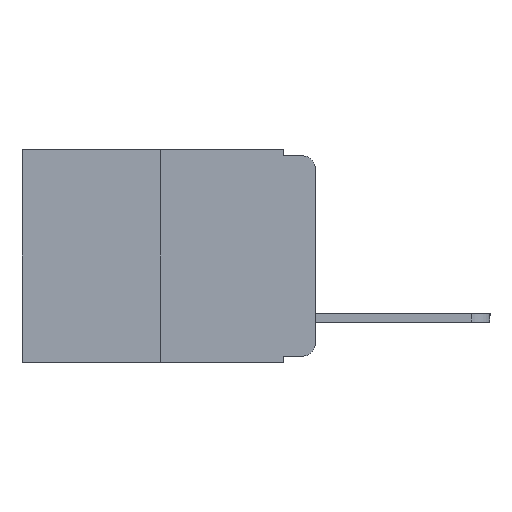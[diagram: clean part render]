
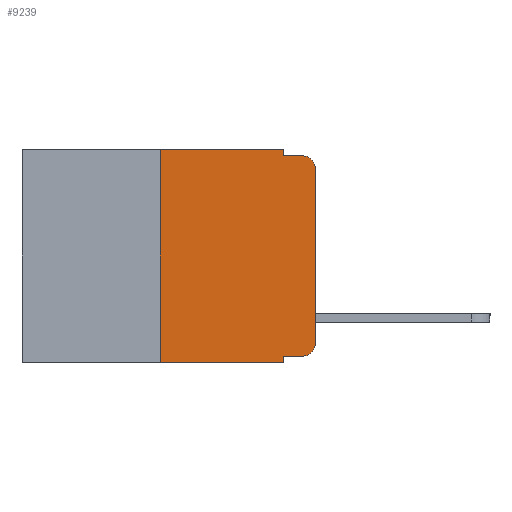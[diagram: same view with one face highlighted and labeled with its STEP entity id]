
A CAD part, left-side view. The second image highlights one B-rep face of the part: STEP entity #9239.
In plain terms, the highlighted planar face has unit normal (-1, 0, 0).
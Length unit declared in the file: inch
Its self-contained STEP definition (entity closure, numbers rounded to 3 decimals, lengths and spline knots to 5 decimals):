
#106 = CARTESIAN_POINT ( 'NONE',  ( 0., 0.473, 0. ) ) ;
#136 = DIRECTION ( 'NONE',  ( 0., 0., -1. ) ) ;
#495 = ORIENTED_EDGE ( 'NONE', *, *, #8389, .T. ) ;
#708 = CARTESIAN_POINT ( 'NONE',  ( 0., 0.02, -0.01 ) ) ;
#1027 = LINE ( 'NONE', #1408, #10063 ) ;
#1173 = DIRECTION ( 'NONE',  ( -1., 0., 0. ) ) ;
#1180 = VERTEX_POINT ( 'NONE', #7032 ) ;
#1190 = CARTESIAN_POINT ( 'NONE',  ( 0., 0.25, 0. ) ) ;
#1201 = CARTESIAN_POINT ( 'NONE',  ( 0., 0.02, -0.313 ) ) ;
#1278 = VERTEX_POINT ( 'NONE', #7676 ) ;
#1378 = CARTESIAN_POINT ( 'NONE',  ( 0., 0.02, -0.03 ) ) ;
#1408 = CARTESIAN_POINT ( 'NONE',  ( 0., 0.473, -0.343 ) ) ;
#1604 = CARTESIAN_POINT ( 'NONE',  ( 0., 0.051, -0.333 ) ) ;
#1689 = DIRECTION ( 'NONE',  ( 0., -1., 0. ) ) ;
#2374 = DIRECTION ( 'NONE',  ( 0., 0., -1. ) ) ;
#2413 = DIRECTION ( 'NONE',  ( 0., -1., 0. ) ) ;
#3088 = ORIENTED_EDGE ( 'NONE', *, *, #10665, .T. ) ;
#3316 = VERTEX_POINT ( 'NONE', #7626 ) ;
#3732 = LINE ( 'NONE', #106, #8022 ) ;
#3818 = EDGE_CURVE ( 'NONE', #10033, #6975, #5031, .T. ) ;
#3880 = CARTESIAN_POINT ( 'NONE',  ( 0., 0.051, -0.333 ) ) ;
#4171 = VERTEX_POINT ( 'NONE', #3880 ) ;
#4238 = DIRECTION ( 'NONE',  ( 0., 0., -1. ) ) ;
#4315 = VECTOR ( 'NONE', #7497, 39.37008 ) ;
#4344 = CARTESIAN_POINT ( 'NONE',  ( 0., 0.25, 0. ) ) ;
#4389 = AXIS2_PLACEMENT_3D ( 'NONE', #4956, #5806, #136 ) ;
#4413 = EDGE_CURVE ( 'NONE', #4171, #10033, #9331, .T. ) ;
#4479 = CARTESIAN_POINT ( 'NONE',  ( 0., 0.051, -0.01 ) ) ;
#4587 = VERTEX_POINT ( 'NONE', #708 ) ;
#4602 = ORIENTED_EDGE ( 'NONE', *, *, #6138, .F. ) ;
#4956 = CARTESIAN_POINT ( 'NONE',  ( 0., 0.473, 0. ) ) ;
#5009 = EDGE_CURVE ( 'NONE', #4171, #1180, #8808, .T. ) ;
#5010 = DIRECTION ( 'NONE',  ( 0., 0., 1. ) ) ;
#5012 = VERTEX_POINT ( 'NONE', #6206 ) ;
#5031 = CIRCLE ( 'NONE', #10215, 0.02 ) ;
#5133 = CARTESIAN_POINT ( 'NONE',  ( 0., 0.051, -0.01 ) ) ;
#5422 = CARTESIAN_POINT ( 'NONE',  ( 0., 0.051, 0. ) ) ;
#5554 = ORIENTED_EDGE ( 'NONE', *, *, #4413, .T. ) ;
#5568 = ORIENTED_EDGE ( 'NONE', *, *, #3818, .T. ) ;
#5593 = ORIENTED_EDGE ( 'NONE', *, *, #10524, .T. ) ;
#5806 = DIRECTION ( 'NONE',  ( 1., 0., 0. ) ) ;
#5978 = DIRECTION ( 'NONE',  ( 0., -1., 0. ) ) ;
#6038 = VECTOR ( 'NONE', #8786, 39.37008 ) ;
#6138 = EDGE_CURVE ( 'NONE', #5012, #7061, #8785, .T. ) ;
#6206 = CARTESIAN_POINT ( 'NONE',  ( 0., 0.25, -0.343 ) ) ;
#6260 = CARTESIAN_POINT ( 'NONE',  ( 0., 0.051, 0. ) ) ;
#6297 = LINE ( 'NONE', #5133, #10385 ) ;
#6631 = VECTOR ( 'NONE', #9207, 39.37008 ) ;
#6800 = EDGE_CURVE ( 'NONE', #7061, #1278, #3732, .T. ) ;
#6876 = ORIENTED_EDGE ( 'NONE', *, *, #7270, .F. ) ;
#6975 = VERTEX_POINT ( 'NONE', #10007 ) ;
#7007 = ORIENTED_EDGE ( 'NONE', *, *, #5009, .F. ) ;
#7032 = CARTESIAN_POINT ( 'NONE',  ( 0., 0.051, -0.343 ) ) ;
#7061 = VERTEX_POINT ( 'NONE', #4344 ) ;
#7270 = EDGE_CURVE ( 'NONE', #1278, #9590, #8267, .T. ) ;
#7497 = DIRECTION ( 'NONE',  ( 0., 0., 1. ) ) ;
#7626 = CARTESIAN_POINT ( 'NONE',  ( 0., 0., -0.03 ) ) ;
#7643 = DIRECTION ( 'NONE',  ( -1., 0., 0. ) ) ;
#7676 = CARTESIAN_POINT ( 'NONE',  ( 0., 0.051, 0. ) ) ;
#7762 = EDGE_LOOP ( 'NONE', ( #5593, #495, #11169, #6876, #11032, #4602, #3088, #7007, #5554, #5568 ) ) ;
#7846 = EDGE_CURVE ( 'NONE', #9590, #4587, #6297, .T. ) ;
#8022 = VECTOR ( 'NONE', #9876, 39.37008 ) ;
#8267 = LINE ( 'NONE', #5422, #6038 ) ;
#8389 = EDGE_CURVE ( 'NONE', #3316, #4587, #11236, .T. ) ;
#8472 = FACE_OUTER_BOUND ( 'NONE', #7762, .T. ) ;
#8785 = LINE ( 'NONE', #1190, #4315 ) ;
#8786 = DIRECTION ( 'NONE',  ( 0., 0., -1. ) ) ;
#8808 = LINE ( 'NONE', #6260, #6631 ) ;
#9201 = LINE ( 'NONE', #9959, #11066 ) ;
#9207 = DIRECTION ( 'NONE',  ( 0., 0., -1. ) ) ;
#9239 = ADVANCED_FACE ( 'NONE', ( #8472 ), #9900, .F. ) ;
#9331 = LINE ( 'NONE', #1604, #11193 ) ;
#9590 = VERTEX_POINT ( 'NONE', #4479 ) ;
#9691 = AXIS2_PLACEMENT_3D ( 'NONE', #1378, #7643, #2374 ) ;
#9876 = DIRECTION ( 'NONE',  ( 0., -1., 0. ) ) ;
#9900 = PLANE ( 'NONE',  #4389 ) ;
#9959 = CARTESIAN_POINT ( 'NONE',  ( 0., 0., 0. ) ) ;
#10007 = CARTESIAN_POINT ( 'NONE',  ( 0., 0., -0.313 ) ) ;
#10033 = VERTEX_POINT ( 'NONE', #11043 ) ;
#10063 = VECTOR ( 'NONE', #2413, 39.37008 ) ;
#10215 = AXIS2_PLACEMENT_3D ( 'NONE', #1201, #1173, #4238 ) ;
#10385 = VECTOR ( 'NONE', #5978, 39.37008 ) ;
#10524 = EDGE_CURVE ( 'NONE', #6975, #3316, #9201, .T. ) ;
#10665 = EDGE_CURVE ( 'NONE', #5012, #1180, #1027, .T. ) ;
#11032 = ORIENTED_EDGE ( 'NONE', *, *, #6800, .F. ) ;
#11043 = CARTESIAN_POINT ( 'NONE',  ( 0., 0.02, -0.333 ) ) ;
#11066 = VECTOR ( 'NONE', #5010, 39.37008 ) ;
#11169 = ORIENTED_EDGE ( 'NONE', *, *, #7846, .F. ) ;
#11193 = VECTOR ( 'NONE', #1689, 39.37008 ) ;
#11236 = CIRCLE ( 'NONE', #9691, 0.02 ) ;
